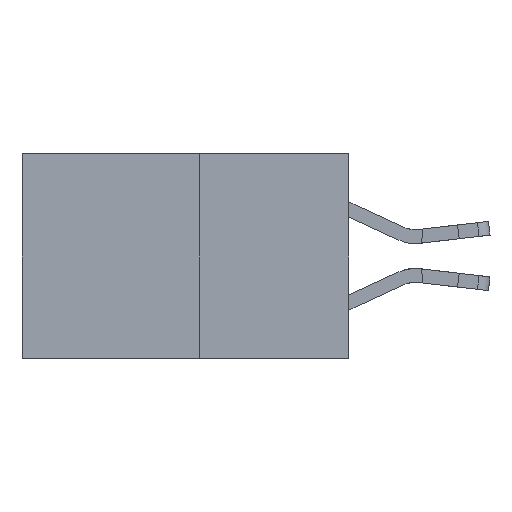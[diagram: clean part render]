
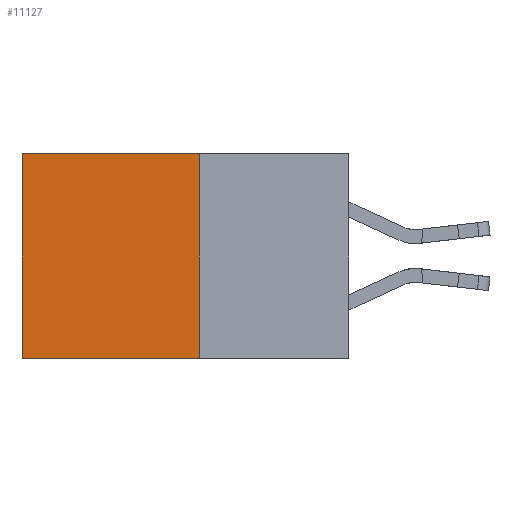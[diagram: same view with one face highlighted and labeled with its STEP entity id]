
A CAD part, left-side view. The second image highlights one B-rep face of the part: STEP entity #11127.
In plain terms, the highlighted planar face has unit normal (-1, 0, 0).
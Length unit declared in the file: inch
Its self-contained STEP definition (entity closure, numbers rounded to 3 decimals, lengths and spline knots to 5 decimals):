
#237 = ORIENTED_EDGE ( 'NONE', *, *, #12258, .F. ) ;
#1097 = CARTESIAN_POINT ( 'NONE',  ( 0.277, 0.27, -0.37 ) ) ;
#1485 = PLANE ( 'NONE',  #26876 ) ;
#1984 = ORIENTED_EDGE ( 'NONE', *, *, #24159, .F. ) ;
#3556 = DIRECTION ( 'NONE',  ( 0., 1., 0. ) ) ;
#3654 = CARTESIAN_POINT ( 'NONE',  ( 0.277, 0.59, -0.37 ) ) ;
#3700 = VECTOR ( 'NONE', #25291, 39.37008 ) ;
#3739 = EDGE_CURVE ( 'NONE', #16312, #25694, #17321, .T. ) ;
#3928 = CARTESIAN_POINT ( 'NONE',  ( 0.277, 0.27, -0.37 ) ) ;
#4063 = FACE_OUTER_BOUND ( 'NONE', #9636, .T. ) ;
#5109 = VECTOR ( 'NONE', #3556, 39.37008 ) ;
#6146 = CARTESIAN_POINT ( 'NONE',  ( 0.277, 0.59, 0. ) ) ;
#7149 = CARTESIAN_POINT ( 'NONE',  ( 0.277, 0.27, -0.37 ) ) ;
#9636 = EDGE_LOOP ( 'NONE', ( #12057, #237, #1984, #9915 ) ) ;
#9915 = ORIENTED_EDGE ( 'NONE', *, *, #3739, .T. ) ;
#10361 = EDGE_CURVE ( 'NONE', #25694, #25805, #18853, .T. ) ;
#11127 = ADVANCED_FACE ( 'NONE', ( #4063 ), #1485, .F. ) ;
#11228 = DIRECTION ( 'NONE',  ( 1., 0., 0. ) ) ;
#11550 = LINE ( 'NONE', #1097, #5109 ) ;
#11663 = VECTOR ( 'NONE', #22821, 39.37008 ) ;
#12057 = ORIENTED_EDGE ( 'NONE', *, *, #10361, .T. ) ;
#12258 = EDGE_CURVE ( 'NONE', #25248, #25805, #11550, .T. ) ;
#16116 = CARTESIAN_POINT ( 'NONE',  ( 0.277, 0.59, -0.37 ) ) ;
#16312 = VERTEX_POINT ( 'NONE', #19077 ) ;
#16591 = LINE ( 'NONE', #22891, #3700 ) ;
#17321 = LINE ( 'NONE', #25558, #29201 ) ;
#18853 = LINE ( 'NONE', #3654, #11663 ) ;
#19077 = CARTESIAN_POINT ( 'NONE',  ( 0.277, 0.27, 0. ) ) ;
#22821 = DIRECTION ( 'NONE',  ( 0., 0., -1. ) ) ;
#22891 = CARTESIAN_POINT ( 'NONE',  ( 0.277, 0.27, -0.37 ) ) ;
#24159 = EDGE_CURVE ( 'NONE', #16312, #25248, #16591, .T. ) ;
#24673 = DIRECTION ( 'NONE',  ( 0., 1., 0. ) ) ;
#25248 = VERTEX_POINT ( 'NONE', #7149 ) ;
#25291 = DIRECTION ( 'NONE',  ( 0., 0., -1. ) ) ;
#25558 = CARTESIAN_POINT ( 'NONE',  ( 0.277, 0.27, 0. ) ) ;
#25694 = VERTEX_POINT ( 'NONE', #6146 ) ;
#25805 = VERTEX_POINT ( 'NONE', #16116 ) ;
#26876 = AXIS2_PLACEMENT_3D ( 'NONE', #3928, #11228, #27982 ) ;
#27982 = DIRECTION ( 'NONE',  ( 0., 0., -1. ) ) ;
#29201 = VECTOR ( 'NONE', #24673, 39.37008 ) ;
